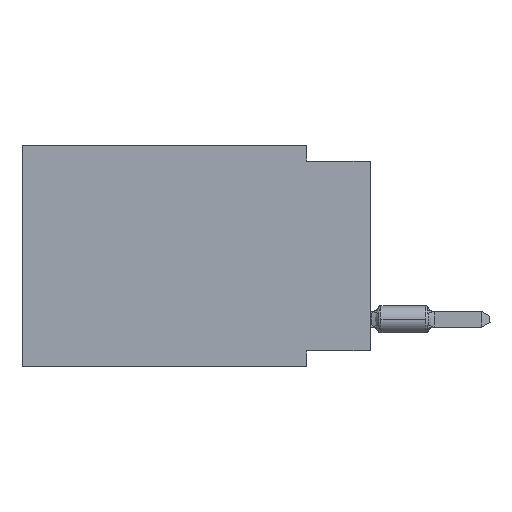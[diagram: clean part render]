
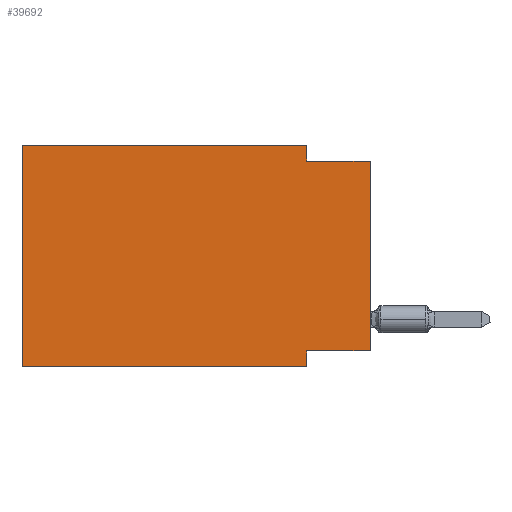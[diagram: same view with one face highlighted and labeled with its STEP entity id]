
A CAD part, left-side view. The second image highlights one B-rep face of the part: STEP entity #39692.
In plain terms, the highlighted planar face has unit normal (-1, 0, 0).
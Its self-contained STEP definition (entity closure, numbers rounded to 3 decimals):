
#68 = DIRECTION ( 'NONE',  ( 0., 0., -1. ) ) ;
#1353 = ORIENTED_EDGE ( 'NONE', *, *, #43195, .F. ) ;
#1784 = LINE ( 'NONE', #35812, #12364 ) ;
#1963 = VECTOR ( 'NONE', #35635, 1000. ) ;
#2088 = EDGE_CURVE ( 'NONE', #8571, #39347, #18130, .T. ) ;
#2618 = ORIENTED_EDGE ( 'NONE', *, *, #46915, .F. ) ;
#3050 = DIRECTION ( 'NONE',  ( 0., 1., 0. ) ) ;
#3154 = CARTESIAN_POINT ( 'NONE',  ( 0., 13.97, 0. ) ) ;
#5200 = LINE ( 'NONE', #38937, #8870 ) ;
#5657 = ORIENTED_EDGE ( 'NONE', *, *, #2088, .F. ) ;
#5869 = DIRECTION ( 'NONE',  ( 0., -1., 0. ) ) ;
#7514 = PLANE ( 'NONE',  #46512 ) ;
#8571 = VERTEX_POINT ( 'NONE', #48810 ) ;
#8870 = VECTOR ( 'NONE', #34755, 1000. ) ;
#11936 = VECTOR ( 'NONE', #68, 1000. ) ;
#12081 = LINE ( 'NONE', #3154, #17706 ) ;
#12364 = VECTOR ( 'NONE', #23768, 1000. ) ;
#17044 = ORIENTED_EDGE ( 'NONE', *, *, #53204, .T. ) ;
#17706 = VECTOR ( 'NONE', #41374, 1000. ) ;
#18130 = LINE ( 'NONE', #26748, #40248 ) ;
#18199 = VECTOR ( 'NONE', #3050, 1000. ) ;
#18205 = VECTOR ( 'NONE', #38822, 1000. ) ;
#18624 = LINE ( 'NONE', #39001, #1963 ) ;
#19169 = EDGE_CURVE ( 'NONE', #41600, #30953, #1784, .T. ) ;
#20848 = ORIENTED_EDGE ( 'NONE', *, *, #19169, .F. ) ;
#21152 = ORIENTED_EDGE ( 'NONE', *, *, #34907, .T. ) ;
#21509 = VERTEX_POINT ( 'NONE', #36483 ) ;
#21804 = CARTESIAN_POINT ( 'NONE',  ( 0., 2.54, 0. ) ) ;
#23746 = CARTESIAN_POINT ( 'NONE',  ( 0., 2.54, 0. ) ) ;
#23768 = DIRECTION ( 'NONE',  ( 0., 0., 1. ) ) ;
#24197 = CARTESIAN_POINT ( 'NONE',  ( 0., 0., -8.255 ) ) ;
#24810 = EDGE_CURVE ( 'NONE', #47476, #8571, #34097, .T. ) ;
#26748 = CARTESIAN_POINT ( 'NONE',  ( 0., 0., -0.635 ) ) ;
#27896 = CARTESIAN_POINT ( 'NONE',  ( 0., 0., -0.635 ) ) ;
#30953 = VERTEX_POINT ( 'NONE', #51421 ) ;
#32293 = DIRECTION ( 'NONE',  ( 1., 0., 0. ) ) ;
#32845 = FACE_OUTER_BOUND ( 'NONE', #45273, .T. ) ;
#34097 = LINE ( 'NONE', #21804, #11936 ) ;
#34755 = DIRECTION ( 'NONE',  ( 0., 0., -1. ) ) ;
#34907 = EDGE_CURVE ( 'NONE', #41600, #21509, #51422, .T. ) ;
#35635 = DIRECTION ( 'NONE',  ( 0., 0., 1. ) ) ;
#35812 = CARTESIAN_POINT ( 'NONE',  ( 0., 13.97, 0. ) ) ;
#36038 = CARTESIAN_POINT ( 'NONE',  ( 0., 2.54, -8.255 ) ) ;
#36053 = EDGE_CURVE ( 'NONE', #30953, #47476, #12081, .T. ) ;
#36483 = CARTESIAN_POINT ( 'NONE',  ( 0., 2.54, -8.89 ) ) ;
#37763 = CARTESIAN_POINT ( 'NONE',  ( 0., 13.97, -8.89 ) ) ;
#38822 = DIRECTION ( 'NONE',  ( 0., -1., 0. ) ) ;
#38937 = CARTESIAN_POINT ( 'NONE',  ( 0., 2.54, -8.89 ) ) ;
#39001 = CARTESIAN_POINT ( 'NONE',  ( 0., 0., 0. ) ) ;
#39347 = VERTEX_POINT ( 'NONE', #27896 ) ;
#39460 = ORIENTED_EDGE ( 'NONE', *, *, #24810, .F. ) ;
#39692 = ADVANCED_FACE ( 'NONE', ( #32845 ), #7514, .F. ) ;
#40248 = VECTOR ( 'NONE', #5869, 1000. ) ;
#41242 = CARTESIAN_POINT ( 'NONE',  ( 0., 13.97, 0. ) ) ;
#41374 = DIRECTION ( 'NONE',  ( 0., -1., 0. ) ) ;
#41600 = VERTEX_POINT ( 'NONE', #37763 ) ;
#41804 = LINE ( 'NONE', #24197, #18199 ) ;
#43195 = EDGE_CURVE ( 'NONE', #45246, #54824, #41804, .T. ) ;
#45246 = VERTEX_POINT ( 'NONE', #51084 ) ;
#45271 = ORIENTED_EDGE ( 'NONE', *, *, #36053, .F. ) ;
#45273 = EDGE_LOOP ( 'NONE', ( #17044, #5657, #39460, #45271, #20848, #21152, #2618, #1353 ) ) ;
#45439 = DIRECTION ( 'NONE',  ( 0., 0., -1. ) ) ;
#46512 = AXIS2_PLACEMENT_3D ( 'NONE', #41242, #32293, #45439 ) ;
#46915 = EDGE_CURVE ( 'NONE', #54824, #21509, #5200, .T. ) ;
#47222 = CARTESIAN_POINT ( 'NONE',  ( 0., 13.97, -8.89 ) ) ;
#47476 = VERTEX_POINT ( 'NONE', #23746 ) ;
#48810 = CARTESIAN_POINT ( 'NONE',  ( 0., 2.54, -0.635 ) ) ;
#51084 = CARTESIAN_POINT ( 'NONE',  ( 0., 0., -8.255 ) ) ;
#51421 = CARTESIAN_POINT ( 'NONE',  ( 0., 13.97, 0. ) ) ;
#51422 = LINE ( 'NONE', #47222, #18205 ) ;
#53204 = EDGE_CURVE ( 'NONE', #45246, #39347, #18624, .T. ) ;
#54824 = VERTEX_POINT ( 'NONE', #36038 ) ;
